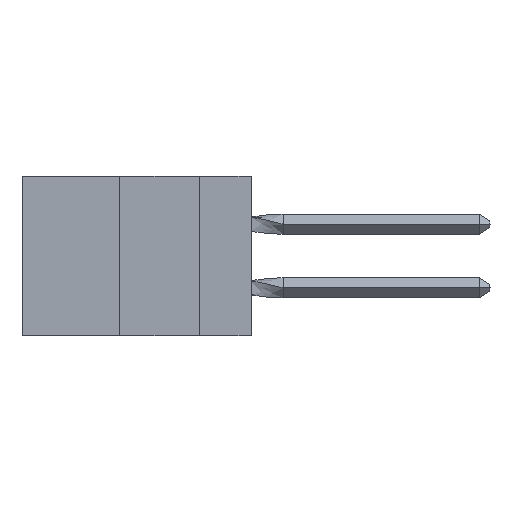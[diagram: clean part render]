
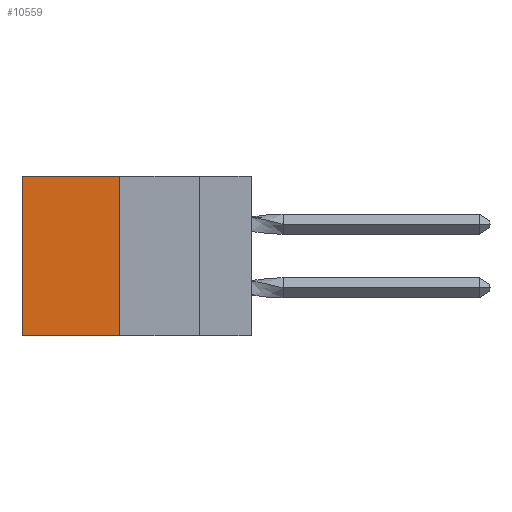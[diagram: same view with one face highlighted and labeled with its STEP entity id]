
A CAD part, left-side view. The second image highlights one B-rep face of the part: STEP entity #10559.
In plain terms, the highlighted planar face has unit normal (-1, 0, 0).
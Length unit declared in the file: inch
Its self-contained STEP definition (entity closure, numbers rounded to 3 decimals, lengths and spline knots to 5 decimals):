
#1151 = CARTESIAN_POINT ( 'NONE',  ( 0.305, 0.72, 0. ) ) ;
#1604 = EDGE_LOOP ( 'NONE', ( #6130, #8044, #9544, #5900 ) ) ;
#2231 = AXIS2_PLACEMENT_3D ( 'NONE', #3866, #18524, #3619 ) ;
#3069 = CARTESIAN_POINT ( 'NONE',  ( 0.305, 0.413, -0.5 ) ) ;
#3252 = EDGE_CURVE ( 'NONE', #4378, #4217, #11453, .T. ) ;
#3619 = DIRECTION ( 'NONE',  ( 0., 0., -1. ) ) ;
#3866 = CARTESIAN_POINT ( 'NONE',  ( 0.305, 0.413, -0.5 ) ) ;
#4217 = VERTEX_POINT ( 'NONE', #3069 ) ;
#4378 = VERTEX_POINT ( 'NONE', #7445 ) ;
#5900 = ORIENTED_EDGE ( 'NONE', *, *, #11286, .T. ) ;
#5902 = DIRECTION ( 'NONE',  ( 0., 0., -1. ) ) ;
#6130 = ORIENTED_EDGE ( 'NONE', *, *, #10337, .T. ) ;
#6222 = DIRECTION ( 'NONE',  ( 0., 1., 0. ) ) ;
#6535 = DIRECTION ( 'NONE',  ( 0., 1., 0. ) ) ;
#6748 = PLANE ( 'NONE',  #2231 ) ;
#7445 = CARTESIAN_POINT ( 'NONE',  ( 0.305, 0.413, 0. ) ) ;
#7596 = VECTOR ( 'NONE', #13370, 39.37008 ) ;
#7941 = CARTESIAN_POINT ( 'NONE',  ( 0.305, 0.72, -0.5 ) ) ;
#8044 = ORIENTED_EDGE ( 'NONE', *, *, #13330, .F. ) ;
#8917 = LINE ( 'NONE', #11095, #13736 ) ;
#9171 = VECTOR ( 'NONE', #5902, 39.37008 ) ;
#9544 = ORIENTED_EDGE ( 'NONE', *, *, #3252, .F. ) ;
#9648 = FACE_OUTER_BOUND ( 'NONE', #1604, .T. ) ;
#10079 = VERTEX_POINT ( 'NONE', #7941 ) ;
#10337 = EDGE_CURVE ( 'NONE', #17480, #10079, #18403, .T. ) ;
#10559 = ADVANCED_FACE ( 'NONE', ( #9648 ), #6748, .F. ) ;
#11095 = CARTESIAN_POINT ( 'NONE',  ( 0.305, 0.413, 0. ) ) ;
#11286 = EDGE_CURVE ( 'NONE', #4378, #17480, #8917, .T. ) ;
#11453 = LINE ( 'NONE', #14706, #9171 ) ;
#12478 = LINE ( 'NONE', #15012, #15439 ) ;
#13330 = EDGE_CURVE ( 'NONE', #4217, #10079, #12478, .T. ) ;
#13370 = DIRECTION ( 'NONE',  ( 0., 0., -1. ) ) ;
#13736 = VECTOR ( 'NONE', #6535, 39.37008 ) ;
#14706 = CARTESIAN_POINT ( 'NONE',  ( 0.305, 0.413, -0.5 ) ) ;
#15012 = CARTESIAN_POINT ( 'NONE',  ( 0.305, 0.413, -0.5 ) ) ;
#15439 = VECTOR ( 'NONE', #6222, 39.37008 ) ;
#16445 = CARTESIAN_POINT ( 'NONE',  ( 0.305, 0.72, -0.5 ) ) ;
#17480 = VERTEX_POINT ( 'NONE', #1151 ) ;
#18403 = LINE ( 'NONE', #16445, #7596 ) ;
#18524 = DIRECTION ( 'NONE',  ( 1., 0., 0. ) ) ;
